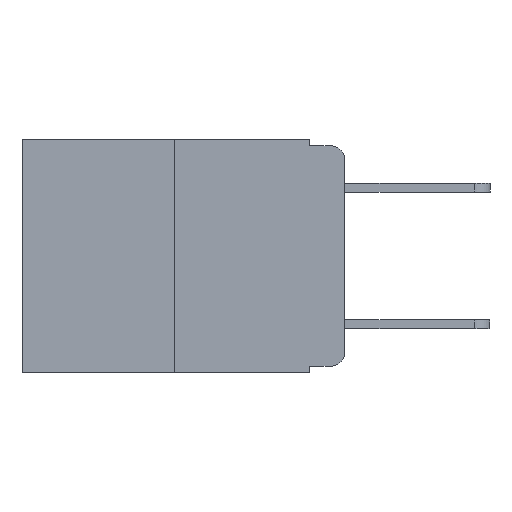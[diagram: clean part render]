
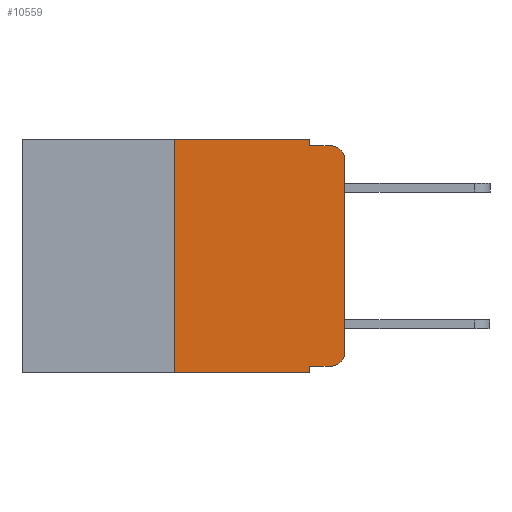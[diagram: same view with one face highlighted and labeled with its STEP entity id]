
A CAD part, left-side view. The second image highlights one B-rep face of the part: STEP entity #10559.
In plain terms, the highlighted planar face has unit normal (-1, 0, 0).
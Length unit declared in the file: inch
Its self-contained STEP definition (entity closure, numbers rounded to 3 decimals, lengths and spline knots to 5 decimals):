
#855 = EDGE_CURVE ( 'NONE', #13629, #12717, #1338, .T. ) ;
#1199 = ORIENTED_EDGE ( 'NONE', *, *, #2893, .F. ) ;
#1224 = VECTOR ( 'NONE', #16253, 39.37008 ) ;
#1338 = CIRCLE ( 'NONE', #10740, 0.02 ) ;
#1519 = DIRECTION ( 'NONE',  ( 0., 0., 1. ) ) ;
#2042 = EDGE_CURVE ( 'NONE', #13816, #15612, #19231, .T. ) ;
#2079 = CARTESIAN_POINT ( 'NONE',  ( 0., 0.25, 0. ) ) ;
#2516 = EDGE_CURVE ( 'NONE', #6923, #12717, #13907, .T. ) ;
#2544 = VERTEX_POINT ( 'NONE', #3701 ) ;
#2818 = CARTESIAN_POINT ( 'NONE',  ( 0., 0., -0.313 ) ) ;
#2821 = ORIENTED_EDGE ( 'NONE', *, *, #2829, .F. ) ;
#2829 = EDGE_CURVE ( 'NONE', #4992, #10447, #14347, .T. ) ;
#2891 = DIRECTION ( 'NONE',  ( -1., 0., 0. ) ) ;
#2893 = EDGE_CURVE ( 'NONE', #15612, #6923, #4710, .T. ) ;
#3169 = VERTEX_POINT ( 'NONE', #14277 ) ;
#3511 = PLANE ( 'NONE',  #3671 ) ;
#3648 = CARTESIAN_POINT ( 'NONE',  ( 0., 0.051, -0.01 ) ) ;
#3671 = AXIS2_PLACEMENT_3D ( 'NONE', #14841, #5243, #16216 ) ;
#3691 = CARTESIAN_POINT ( 'NONE',  ( 0., 0.25, 0. ) ) ;
#3701 = CARTESIAN_POINT ( 'NONE',  ( 0., 0.02, -0.333 ) ) ;
#3860 = ORIENTED_EDGE ( 'NONE', *, *, #8942, .T. ) ;
#4078 = DIRECTION ( 'NONE',  ( 0., -1., 0. ) ) ;
#4354 = EDGE_CURVE ( 'NONE', #3169, #13816, #17299, .T. ) ;
#4710 = LINE ( 'NONE', #18833, #12934 ) ;
#4729 = VECTOR ( 'NONE', #4078, 39.37008 ) ;
#4774 = VERTEX_POINT ( 'NONE', #2818 ) ;
#4992 = VERTEX_POINT ( 'NONE', #17167 ) ;
#4995 = EDGE_CURVE ( 'NONE', #4992, #2544, #12400, .T. ) ;
#5204 = ORIENTED_EDGE ( 'NONE', *, *, #2516, .F. ) ;
#5243 = DIRECTION ( 'NONE',  ( 1., 0., 0. ) ) ;
#5437 = ORIENTED_EDGE ( 'NONE', *, *, #7835, .T. ) ;
#6923 = VERTEX_POINT ( 'NONE', #3648 ) ;
#7245 = DIRECTION ( 'NONE',  ( -1., 0., 0. ) ) ;
#7315 = ORIENTED_EDGE ( 'NONE', *, *, #4995, .T. ) ;
#7468 = VECTOR ( 'NONE', #19740, 39.37008 ) ;
#7506 = VECTOR ( 'NONE', #16003, 39.37008 ) ;
#7835 = EDGE_CURVE ( 'NONE', #3169, #10447, #18512, .T. ) ;
#8203 = CARTESIAN_POINT ( 'NONE',  ( 0., 0.02, -0.01 ) ) ;
#8942 = EDGE_CURVE ( 'NONE', #2544, #4774, #12293, .T. ) ;
#9291 = ORIENTED_EDGE ( 'NONE', *, *, #855, .T. ) ;
#9631 = DIRECTION ( 'NONE',  ( 0., 0., 1. ) ) ;
#9660 = VECTOR ( 'NONE', #9631, 39.37008 ) ;
#9822 = EDGE_CURVE ( 'NONE', #4774, #13629, #16965, .T. ) ;
#9889 = CARTESIAN_POINT ( 'NONE',  ( 0., 0.473, -0.343 ) ) ;
#10447 = VERTEX_POINT ( 'NONE', #19845 ) ;
#10559 = ADVANCED_FACE ( 'NONE', ( #18625 ), #3511, .F. ) ;
#10740 = AXIS2_PLACEMENT_3D ( 'NONE', #11181, #7245, #16738 ) ;
#11181 = CARTESIAN_POINT ( 'NONE',  ( 0., 0.02, -0.03 ) ) ;
#12293 = CIRCLE ( 'NONE', #19991, 0.02 ) ;
#12400 = LINE ( 'NONE', #16695, #7506 ) ;
#12664 = ORIENTED_EDGE ( 'NONE', *, *, #9822, .T. ) ;
#12717 = VERTEX_POINT ( 'NONE', #8203 ) ;
#12822 = CARTESIAN_POINT ( 'NONE',  ( 0., 0.02, -0.313 ) ) ;
#12934 = VECTOR ( 'NONE', #18794, 39.37008 ) ;
#13629 = VERTEX_POINT ( 'NONE', #17369 ) ;
#13816 = VERTEX_POINT ( 'NONE', #2079 ) ;
#13907 = LINE ( 'NONE', #19927, #4729 ) ;
#14277 = CARTESIAN_POINT ( 'NONE',  ( 0., 0.25, -0.343 ) ) ;
#14320 = DIRECTION ( 'NONE',  ( 0., 0., -1. ) ) ;
#14347 = LINE ( 'NONE', #16188, #1224 ) ;
#14743 = ORIENTED_EDGE ( 'NONE', *, *, #4354, .F. ) ;
#14841 = CARTESIAN_POINT ( 'NONE',  ( 0., 0.473, 0. ) ) ;
#15612 = VERTEX_POINT ( 'NONE', #19657 ) ;
#15656 = VECTOR ( 'NONE', #19567, 39.37008 ) ;
#15989 = VECTOR ( 'NONE', #1519, 39.37008 ) ;
#16003 = DIRECTION ( 'NONE',  ( 0., -1., 0. ) ) ;
#16188 = CARTESIAN_POINT ( 'NONE',  ( 0., 0.051, 0. ) ) ;
#16216 = DIRECTION ( 'NONE',  ( 0., 0., -1. ) ) ;
#16253 = DIRECTION ( 'NONE',  ( 0., 0., -1. ) ) ;
#16695 = CARTESIAN_POINT ( 'NONE',  ( 0., 0.051, -0.333 ) ) ;
#16738 = DIRECTION ( 'NONE',  ( 0., 0., -1. ) ) ;
#16965 = LINE ( 'NONE', #18288, #9660 ) ;
#17167 = CARTESIAN_POINT ( 'NONE',  ( 0., 0.051, -0.333 ) ) ;
#17299 = LINE ( 'NONE', #3691, #15989 ) ;
#17369 = CARTESIAN_POINT ( 'NONE',  ( 0., 0., -0.03 ) ) ;
#17776 = EDGE_LOOP ( 'NONE', ( #12664, #9291, #5204, #1199, #17961, #14743, #5437, #2821, #7315, #3860 ) ) ;
#17961 = ORIENTED_EDGE ( 'NONE', *, *, #2042, .F. ) ;
#18288 = CARTESIAN_POINT ( 'NONE',  ( 0., 0., 0. ) ) ;
#18512 = LINE ( 'NONE', #9889, #7468 ) ;
#18625 = FACE_OUTER_BOUND ( 'NONE', #17776, .T. ) ;
#18794 = DIRECTION ( 'NONE',  ( 0., 0., -1. ) ) ;
#18833 = CARTESIAN_POINT ( 'NONE',  ( 0., 0.051, 0. ) ) ;
#19231 = LINE ( 'NONE', #19555, #15656 ) ;
#19555 = CARTESIAN_POINT ( 'NONE',  ( 0., 0.473, 0. ) ) ;
#19567 = DIRECTION ( 'NONE',  ( 0., -1., 0. ) ) ;
#19657 = CARTESIAN_POINT ( 'NONE',  ( 0., 0.051, 0. ) ) ;
#19740 = DIRECTION ( 'NONE',  ( 0., -1., 0. ) ) ;
#19845 = CARTESIAN_POINT ( 'NONE',  ( 0., 0.051, -0.343 ) ) ;
#19927 = CARTESIAN_POINT ( 'NONE',  ( 0., 0.051, -0.01 ) ) ;
#19991 = AXIS2_PLACEMENT_3D ( 'NONE', #12822, #2891, #14320 ) ;
